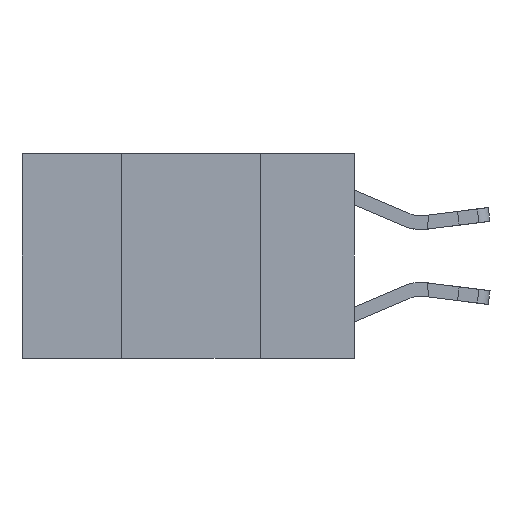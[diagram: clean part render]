
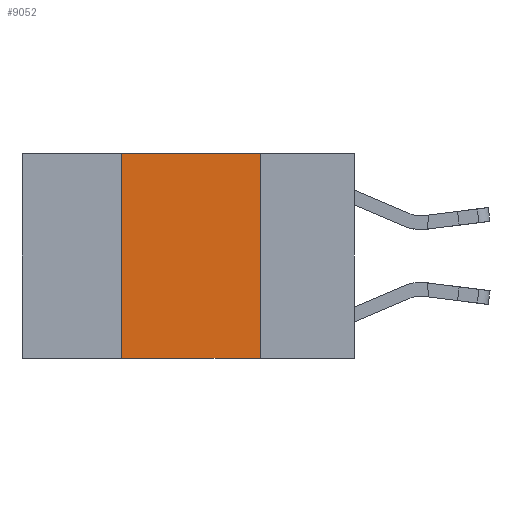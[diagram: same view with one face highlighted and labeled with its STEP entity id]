
A CAD part, left-side view. The second image highlights one B-rep face of the part: STEP entity #9052.
In plain terms, the highlighted planar face has unit normal (-1, 0, 0).
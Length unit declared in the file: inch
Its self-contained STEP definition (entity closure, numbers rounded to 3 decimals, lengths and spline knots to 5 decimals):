
#817 = CARTESIAN_POINT ( 'NONE',  ( 0., 0.17, 0. ) ) ;
#1837 = VERTEX_POINT ( 'NONE', #817 ) ;
#3014 = AXIS2_PLACEMENT_3D ( 'NONE', #18307, #20329, #8078 ) ;
#3942 = PLANE ( 'NONE',  #3014 ) ;
#3999 = CARTESIAN_POINT ( 'NONE',  ( 0., 0.42, 0. ) ) ;
#5745 = VECTOR ( 'NONE', #20837, 39.37008 ) ;
#6082 = EDGE_CURVE ( 'NONE', #11049, #26104, #22056, .T. ) ;
#6621 = DIRECTION ( 'NONE',  ( 0., -1., 0. ) ) ;
#7836 = FACE_OUTER_BOUND ( 'NONE', #18812, .T. ) ;
#8078 = DIRECTION ( 'NONE',  ( 0., 0., -1. ) ) ;
#8134 = VECTOR ( 'NONE', #15082, 39.37008 ) ;
#8688 = ORIENTED_EDGE ( 'NONE', *, *, #12127, .T. ) ;
#8846 = CARTESIAN_POINT ( 'NONE',  ( 0., 0.17, 0. ) ) ;
#9052 = ADVANCED_FACE ( 'NONE', ( #7836 ), #3942, .F. ) ;
#9429 = LINE ( 'NONE', #8846, #8134 ) ;
#9905 = EDGE_CURVE ( 'NONE', #26104, #1837, #19696, .T. ) ;
#11049 = VERTEX_POINT ( 'NONE', #19586 ) ;
#11098 = CARTESIAN_POINT ( 'NONE',  ( 0., 0.6, 0. ) ) ;
#12127 = EDGE_CURVE ( 'NONE', #11049, #17394, #17844, .T. ) ;
#15082 = DIRECTION ( 'NONE',  ( 0., 0., -1. ) ) ;
#15586 = VECTOR ( 'NONE', #25250, 39.37008 ) ;
#17394 = VERTEX_POINT ( 'NONE', #19372 ) ;
#17844 = LINE ( 'NONE', #20915, #22552 ) ;
#18307 = CARTESIAN_POINT ( 'NONE',  ( 0., 0.6, 0. ) ) ;
#18812 = EDGE_LOOP ( 'NONE', ( #22113, #22233, #23446, #8688 ) ) ;
#18842 = CARTESIAN_POINT ( 'NONE',  ( 0., 0.42, 0. ) ) ;
#19372 = CARTESIAN_POINT ( 'NONE',  ( 0., 0.17, -0.37 ) ) ;
#19586 = CARTESIAN_POINT ( 'NONE',  ( 0., 0.42, -0.37 ) ) ;
#19696 = LINE ( 'NONE', #11098, #15586 ) ;
#20329 = DIRECTION ( 'NONE',  ( 1., 0., 0. ) ) ;
#20837 = DIRECTION ( 'NONE',  ( 0., 0., 1. ) ) ;
#20915 = CARTESIAN_POINT ( 'NONE',  ( 0., 0.6, -0.37 ) ) ;
#22056 = LINE ( 'NONE', #18842, #5745 ) ;
#22113 = ORIENTED_EDGE ( 'NONE', *, *, #24315, .F. ) ;
#22233 = ORIENTED_EDGE ( 'NONE', *, *, #9905, .F. ) ;
#22552 = VECTOR ( 'NONE', #6621, 39.37008 ) ;
#23446 = ORIENTED_EDGE ( 'NONE', *, *, #6082, .F. ) ;
#24315 = EDGE_CURVE ( 'NONE', #1837, #17394, #9429, .T. ) ;
#25250 = DIRECTION ( 'NONE',  ( 0., -1., 0. ) ) ;
#26104 = VERTEX_POINT ( 'NONE', #3999 ) ;
